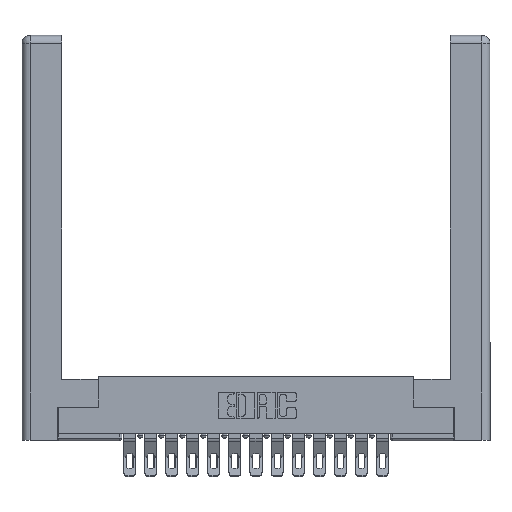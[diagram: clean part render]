
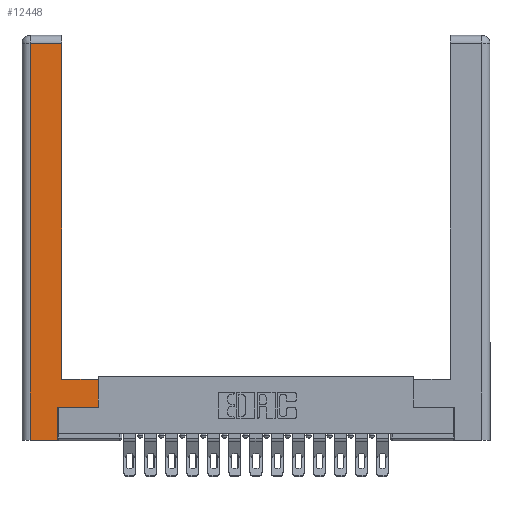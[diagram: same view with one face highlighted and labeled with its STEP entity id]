
A CAD part, top view. The second image highlights one B-rep face of the part: STEP entity #12448.
In plain terms, the highlighted planar face has unit normal (0, 0, 1).
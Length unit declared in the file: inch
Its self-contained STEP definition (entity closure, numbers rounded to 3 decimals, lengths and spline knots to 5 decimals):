
#39 = EDGE_CURVE ( 'NONE', #11317, #2898, #9724, .T. ) ;
#107 = LINE ( 'NONE', #18202, #7585 ) ;
#571 = CARTESIAN_POINT ( 'NONE',  ( 0.565, 0.45, 0. ) ) ;
#726 = CARTESIAN_POINT ( 'NONE',  ( 0.565, 0.245, 0. ) ) ;
#1231 = DIRECTION ( 'NONE',  ( 0., 1., 0. ) ) ;
#1242 = DIRECTION ( 'NONE',  ( 0., -1., 0. ) ) ;
#1302 = CARTESIAN_POINT ( 'NONE',  ( 0.0615, 2.94, 0. ) ) ;
#1471 = LINE ( 'NONE', #9936, #11594 ) ;
#1481 = CARTESIAN_POINT ( 'NONE',  ( 0.295, 0.45, 0. ) ) ;
#1531 = CARTESIAN_POINT ( 'NONE',  ( 0.265, 0., 0. ) ) ;
#1732 = ORIENTED_EDGE ( 'NONE', *, *, #16257, .T. ) ;
#1764 = LINE ( 'NONE', #12482, #4856 ) ;
#2895 = EDGE_CURVE ( 'NONE', #11658, #9242, #1471, .T. ) ;
#2898 = VERTEX_POINT ( 'NONE', #12869 ) ;
#2909 = VECTOR ( 'NONE', #12822, 39.37008 ) ;
#2987 = DIRECTION ( 'NONE',  ( -1., 0., 0. ) ) ;
#2993 = VECTOR ( 'NONE', #5500, 39.37008 ) ;
#3844 = ORIENTED_EDGE ( 'NONE', *, *, #15021, .T. ) ;
#4408 = AXIS2_PLACEMENT_3D ( 'NONE', #12998, #7289, #2987 ) ;
#4544 = EDGE_CURVE ( 'NONE', #14907, #8215, #1764, .T. ) ;
#4856 = VECTOR ( 'NONE', #1242, 39.37008 ) ;
#4925 = VECTOR ( 'NONE', #1231, 39.37008 ) ;
#4950 = EDGE_LOOP ( 'NONE', ( #1732, #10895, #10650, #15440, #6528, #7013, #17751, #3844 ) ) ;
#5500 = DIRECTION ( 'NONE',  ( -1., 0., 0. ) ) ;
#5838 = VERTEX_POINT ( 'NONE', #7567 ) ;
#5917 = VECTOR ( 'NONE', #17399, 39.37008 ) ;
#6528 = ORIENTED_EDGE ( 'NONE', *, *, #2895, .T. ) ;
#7013 = ORIENTED_EDGE ( 'NONE', *, *, #12192, .T. ) ;
#7289 = DIRECTION ( 'NONE',  ( 0., 0., -1. ) ) ;
#7567 = CARTESIAN_POINT ( 'NONE',  ( 0.295, 0.45, 0. ) ) ;
#7585 = VECTOR ( 'NONE', #16798, 39.37008 ) ;
#7591 = DIRECTION ( 'NONE',  ( 0., 1., 0. ) ) ;
#7726 = FACE_OUTER_BOUND ( 'NONE', #4950, .T. ) ;
#8051 = EDGE_CURVE ( 'NONE', #15067, #14907, #9628, .T. ) ;
#8215 = VERTEX_POINT ( 'NONE', #12005 ) ;
#9242 = VERTEX_POINT ( 'NONE', #15305 ) ;
#9628 = LINE ( 'NONE', #13067, #5917 ) ;
#9724 = LINE ( 'NONE', #571, #16864 ) ;
#9936 = CARTESIAN_POINT ( 'NONE',  ( 0.265, 0.245, 0. ) ) ;
#9976 = CARTESIAN_POINT ( 'NONE',  ( 0.295, 2.94, 0. ) ) ;
#10058 = DIRECTION ( 'NONE',  ( 0., 1., 0. ) ) ;
#10224 = EDGE_CURVE ( 'NONE', #8215, #11658, #107, .T. ) ;
#10650 = ORIENTED_EDGE ( 'NONE', *, *, #4544, .T. ) ;
#10895 = ORIENTED_EDGE ( 'NONE', *, *, #8051, .T. ) ;
#11317 = VERTEX_POINT ( 'NONE', #726 ) ;
#11594 = VECTOR ( 'NONE', #10058, 39.37008 ) ;
#11658 = VERTEX_POINT ( 'NONE', #1531 ) ;
#12005 = CARTESIAN_POINT ( 'NONE',  ( 0.0615, 0., 0. ) ) ;
#12192 = EDGE_CURVE ( 'NONE', #9242, #11317, #13917, .T. ) ;
#12448 = ADVANCED_FACE ( 'NONE', ( #7726 ), #15766, .F. ) ;
#12482 = CARTESIAN_POINT ( 'NONE',  ( 0.0615, 0., 0. ) ) ;
#12822 = DIRECTION ( 'NONE',  ( 1., 0., 0. ) ) ;
#12869 = CARTESIAN_POINT ( 'NONE',  ( 0.565, 0.45, 0. ) ) ;
#12998 = CARTESIAN_POINT ( 'NONE',  ( 0., 0., 0. ) ) ;
#13067 = CARTESIAN_POINT ( 'NONE',  ( 0.0615, 2.94, 0. ) ) ;
#13917 = LINE ( 'NONE', #17153, #2909 ) ;
#14843 = LINE ( 'NONE', #15430, #4925 ) ;
#14907 = VERTEX_POINT ( 'NONE', #1302 ) ;
#15021 = EDGE_CURVE ( 'NONE', #2898, #5838, #16251, .T. ) ;
#15067 = VERTEX_POINT ( 'NONE', #9976 ) ;
#15305 = CARTESIAN_POINT ( 'NONE',  ( 0.265, 0.245, 0. ) ) ;
#15430 = CARTESIAN_POINT ( 'NONE',  ( 0.295, 3., 0. ) ) ;
#15440 = ORIENTED_EDGE ( 'NONE', *, *, #10224, .T. ) ;
#15766 = PLANE ( 'NONE',  #4408 ) ;
#16251 = LINE ( 'NONE', #1481, #2993 ) ;
#16257 = EDGE_CURVE ( 'NONE', #5838, #15067, #14843, .T. ) ;
#16798 = DIRECTION ( 'NONE',  ( 1., 0., 0. ) ) ;
#16864 = VECTOR ( 'NONE', #7591, 39.37008 ) ;
#17153 = CARTESIAN_POINT ( 'NONE',  ( 0.565, 0.245, 0. ) ) ;
#17399 = DIRECTION ( 'NONE',  ( -1., 0., 0. ) ) ;
#17751 = ORIENTED_EDGE ( 'NONE', *, *, #39, .T. ) ;
#18202 = CARTESIAN_POINT ( 'NONE',  ( 0.265, 0., 0. ) ) ;
